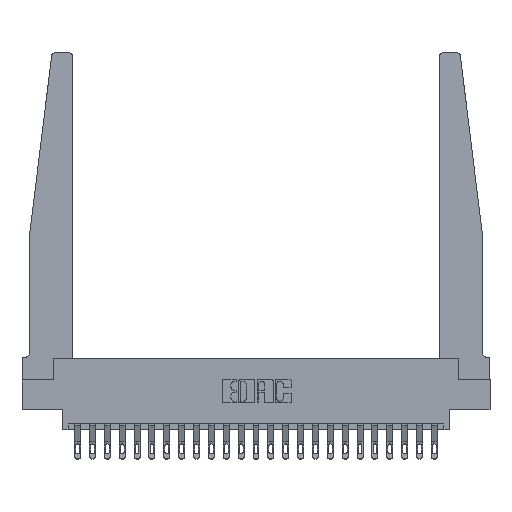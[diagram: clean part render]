
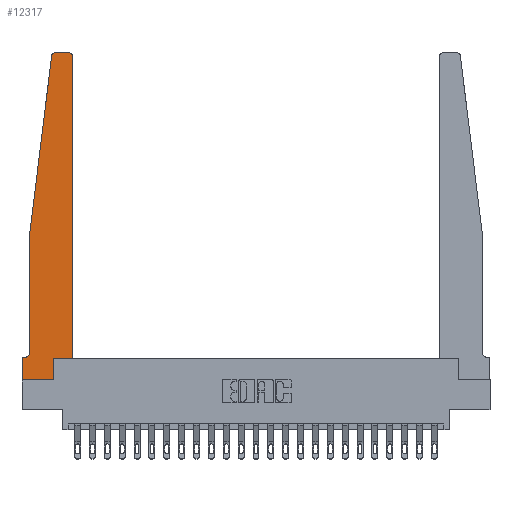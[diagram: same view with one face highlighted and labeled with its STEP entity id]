
A CAD part, top view. The second image highlights one B-rep face of the part: STEP entity #12317.
In plain terms, the highlighted planar face has unit normal (0, 0, 1).
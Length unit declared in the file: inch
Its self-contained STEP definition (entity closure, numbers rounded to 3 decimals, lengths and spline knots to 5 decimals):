
#406 = VECTOR ( 'NONE', #550, 39.37008 ) ;
#550 = DIRECTION ( 'NONE',  ( 0., 1., 0. ) ) ;
#785 = DIRECTION ( 'NONE',  ( 0., 0., 1. ) ) ;
#1792 = CARTESIAN_POINT ( 'NONE',  ( 0.065, 1.25, 0.37 ) ) ;
#2023 = DIRECTION ( 'NONE',  ( 1., 0., 0. ) ) ;
#2062 = EDGE_CURVE ( 'NONE', #15353, #13506, #18029, .T. ) ;
#2152 = DIRECTION ( 'NONE',  ( -1., 0., 0. ) ) ;
#2153 = EDGE_CURVE ( 'NONE', #9950, #8881, #16301, .T. ) ;
#2516 = LINE ( 'NONE', #4321, #21537 ) ;
#3123 = ORIENTED_EDGE ( 'NONE', *, *, #10486, .T. ) ;
#3230 = VERTEX_POINT ( 'NONE', #8947 ) ;
#3648 = DIRECTION ( 'NONE',  ( -1., 0., 0. ) ) ;
#3751 = CIRCLE ( 'NONE', #17978, 0.03 ) ;
#4321 = CARTESIAN_POINT ( 'NONE',  ( 0.425, 0.18, 0.37 ) ) ;
#4405 = DIRECTION ( 'NONE',  ( 0., 1., 0. ) ) ;
#4710 = LINE ( 'NONE', #6056, #406 ) ;
#4841 = ORIENTED_EDGE ( 'NONE', *, *, #7089, .T. ) ;
#5496 = DIRECTION ( 'NONE',  ( -0.122, -0.992, 0. ) ) ;
#5737 = ORIENTED_EDGE ( 'NONE', *, *, #18132, .T. ) ;
#5929 = VECTOR ( 'NONE', #9650, 39.37008 ) ;
#6056 = CARTESIAN_POINT ( 'NONE',  ( 0.2605, 0.18, 0.37 ) ) ;
#6668 = VERTEX_POINT ( 'NONE', #19449 ) ;
#6770 = CARTESIAN_POINT ( 'NONE',  ( 0.425, 0.18, 0.37 ) ) ;
#6839 = CARTESIAN_POINT ( 'NONE',  ( 0., 0., 0.37 ) ) ;
#6968 = FACE_OUTER_BOUND ( 'NONE', #15261, .T. ) ;
#7089 = EDGE_CURVE ( 'NONE', #20671, #14520, #20606, .T. ) ;
#7491 = VECTOR ( 'NONE', #3648, 39.37008 ) ;
#7770 = CARTESIAN_POINT ( 'NONE',  ( 0.065, 1.25, 0.37 ) ) ;
#7876 = CARTESIAN_POINT ( 'NONE',  ( 0.2605, 0., 0.37 ) ) ;
#8152 = PLANE ( 'NONE',  #20808 ) ;
#8513 = CARTESIAN_POINT ( 'NONE',  ( 0.395, 2.75, 0.37 ) ) ;
#8794 = CARTESIAN_POINT ( 'NONE',  ( 0.015, 0.2375, 0.37 ) ) ;
#8880 = CARTESIAN_POINT ( 'NONE',  ( 0.27653, 2.72, 0.37 ) ) ;
#8881 = VERTEX_POINT ( 'NONE', #6770 ) ;
#8947 = CARTESIAN_POINT ( 'NONE',  ( 0.015, 0.1875, 0.37 ) ) ;
#8972 = EDGE_CURVE ( 'NONE', #21671, #15360, #14834, .T. ) ;
#9242 = ORIENTED_EDGE ( 'NONE', *, *, #2153, .T. ) ;
#9323 = CARTESIAN_POINT ( 'NONE',  ( 0.395, 2.72, 0.37 ) ) ;
#9650 = DIRECTION ( 'NONE',  ( 0., -1., 0. ) ) ;
#9891 = CARTESIAN_POINT ( 'NONE',  ( 0.24675, 2.72367, 0.37 ) ) ;
#9950 = VERTEX_POINT ( 'NONE', #22786 ) ;
#10343 = EDGE_CURVE ( 'NONE', #17302, #20671, #21737, .T. ) ;
#10486 = EDGE_CURVE ( 'NONE', #15360, #9950, #4710, .T. ) ;
#10645 = DIRECTION ( 'NONE',  ( -1., 0., 0. ) ) ;
#10725 = DIRECTION ( 'NONE',  ( 1., 0., 0. ) ) ;
#10738 = CARTESIAN_POINT ( 'NONE',  ( 0., 0., 0.37 ) ) ;
#10948 = EDGE_CURVE ( 'NONE', #3230, #6668, #15128, .T. ) ;
#11084 = VECTOR ( 'NONE', #23570, 39.37008 ) ;
#11117 = EDGE_CURVE ( 'NONE', #6668, #21671, #20827, .T. ) ;
#11171 = DIRECTION ( 'NONE',  ( 1., 0., 0. ) ) ;
#11237 = ORIENTED_EDGE ( 'NONE', *, *, #13732, .T. ) ;
#11319 = CARTESIAN_POINT ( 'NONE',  ( 0.425, 0.18, 0.37 ) ) ;
#11864 = CARTESIAN_POINT ( 'NONE',  ( 0., 0.1875, 0.37 ) ) ;
#12221 = VECTOR ( 'NONE', #5496, 39.37008 ) ;
#12317 = ADVANCED_FACE ( 'NONE', ( #6968 ), #8152, .T. ) ;
#12979 = ORIENTED_EDGE ( 'NONE', *, *, #19620, .T. ) ;
#13506 = VERTEX_POINT ( 'NONE', #8513 ) ;
#13705 = DIRECTION ( 'NONE',  ( 0., -1., 0. ) ) ;
#13732 = EDGE_CURVE ( 'NONE', #13506, #19214, #21574, .T. ) ;
#13735 = DIRECTION ( 'NONE',  ( 1., 0., 0. ) ) ;
#14520 = VERTEX_POINT ( 'NONE', #18619 ) ;
#14834 = LINE ( 'NONE', #10738, #11084 ) ;
#15082 = CARTESIAN_POINT ( 'NONE',  ( 0.065, 0.1875, 0.37 ) ) ;
#15128 = LINE ( 'NONE', #15082, #19412 ) ;
#15261 = EDGE_LOOP ( 'NONE', ( #11237, #5737, #16120, #4841, #20136, #16691, #21567, #15274, #3123, #9242, #12979, #16794 ) ) ;
#15274 = ORIENTED_EDGE ( 'NONE', *, *, #8972, .T. ) ;
#15353 = VERTEX_POINT ( 'NONE', #18914 ) ;
#15360 = VERTEX_POINT ( 'NONE', #7876 ) ;
#15518 = AXIS2_PLACEMENT_3D ( 'NONE', #8794, #21634, #10645 ) ;
#15967 = VECTOR ( 'NONE', #13705, 39.37008 ) ;
#16120 = ORIENTED_EDGE ( 'NONE', *, *, #10343, .T. ) ;
#16301 = LINE ( 'NONE', #11319, #21746 ) ;
#16551 = CARTESIAN_POINT ( 'NONE',  ( 0.25, 2.75, 0.37 ) ) ;
#16691 = ORIENTED_EDGE ( 'NONE', *, *, #10948, .T. ) ;
#16794 = ORIENTED_EDGE ( 'NONE', *, *, #2062, .T. ) ;
#17302 = VERTEX_POINT ( 'NONE', #9891 ) ;
#17978 = AXIS2_PLACEMENT_3D ( 'NONE', #8880, #21716, #10725 ) ;
#18029 = CIRCLE ( 'NONE', #18439, 0.03 ) ;
#18119 = EDGE_CURVE ( 'NONE', #14520, #3230, #23327, .T. ) ;
#18132 = EDGE_CURVE ( 'NONE', #19214, #17302, #3751, .T. ) ;
#18439 = AXIS2_PLACEMENT_3D ( 'NONE', #9323, #22153, #11171 ) ;
#18619 = CARTESIAN_POINT ( 'NONE',  ( 0.065, 0.2375, 0.37 ) ) ;
#18914 = CARTESIAN_POINT ( 'NONE',  ( 0.425, 2.72, 0.37 ) ) ;
#19214 = VERTEX_POINT ( 'NONE', #23352 ) ;
#19412 = VECTOR ( 'NONE', #2152, 39.37008 ) ;
#19449 = CARTESIAN_POINT ( 'NONE',  ( 0., 0.1875, 0.37 ) ) ;
#19620 = EDGE_CURVE ( 'NONE', #8881, #15353, #2516, .T. ) ;
#20136 = ORIENTED_EDGE ( 'NONE', *, *, #18119, .T. ) ;
#20606 = LINE ( 'NONE', #7770, #5929 ) ;
#20671 = VERTEX_POINT ( 'NONE', #1792 ) ;
#20808 = AXIS2_PLACEMENT_3D ( 'NONE', #11864, #785, #13735 ) ;
#20827 = LINE ( 'NONE', #22816, #15967 ) ;
#21537 = VECTOR ( 'NONE', #4405, 39.37008 ) ;
#21567 = ORIENTED_EDGE ( 'NONE', *, *, #11117, .T. ) ;
#21574 = LINE ( 'NONE', #16551, #7491 ) ;
#21634 = DIRECTION ( 'NONE',  ( 0., 0., -1. ) ) ;
#21671 = VERTEX_POINT ( 'NONE', #6839 ) ;
#21716 = DIRECTION ( 'NONE',  ( 0., 0., 1. ) ) ;
#21737 = LINE ( 'NONE', #22069, #12221 ) ;
#21746 = VECTOR ( 'NONE', #2023, 39.37008 ) ;
#22069 = CARTESIAN_POINT ( 'NONE',  ( 0.065, 1.25, 0.37 ) ) ;
#22153 = DIRECTION ( 'NONE',  ( 0., 0., 1. ) ) ;
#22786 = CARTESIAN_POINT ( 'NONE',  ( 0.2605, 0.18, 0.37 ) ) ;
#22816 = CARTESIAN_POINT ( 'NONE',  ( 0., 0., 0.37 ) ) ;
#23327 = CIRCLE ( 'NONE', #15518, 0.05 ) ;
#23352 = CARTESIAN_POINT ( 'NONE',  ( 0.27653, 2.75, 0.37 ) ) ;
#23570 = DIRECTION ( 'NONE',  ( 1., 0., 0. ) ) ;
